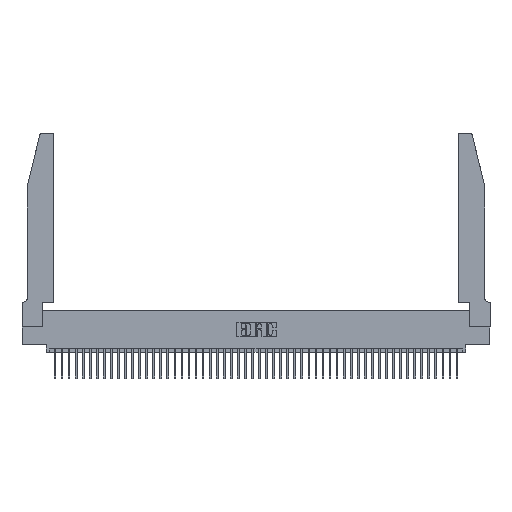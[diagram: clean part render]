
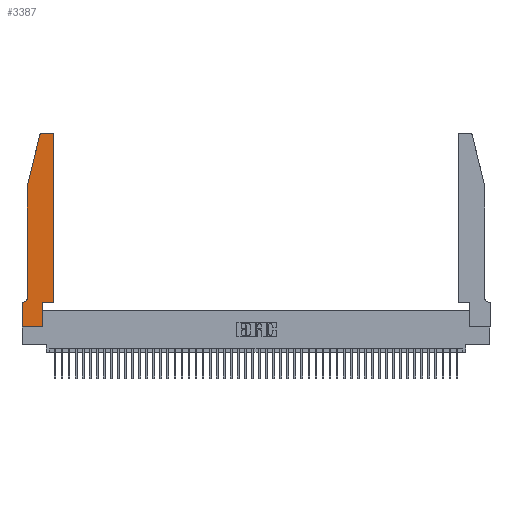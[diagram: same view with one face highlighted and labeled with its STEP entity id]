
A CAD part, top view. The second image highlights one B-rep face of the part: STEP entity #3387.
In plain terms, the highlighted planar face has unit normal (0, 0, 1).
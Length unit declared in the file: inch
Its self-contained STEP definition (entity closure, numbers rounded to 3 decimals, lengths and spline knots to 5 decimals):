
#514 = ORIENTED_EDGE ( 'NONE', *, *, #25352, .T. ) ;
#854 = VECTOR ( 'NONE', #18013, 39.37008 ) ;
#1100 = CARTESIAN_POINT ( 'NONE',  ( 0.0755, 0.42, 0.37 ) ) ;
#1218 = EDGE_CURVE ( 'NONE', #14511, #22834, #33169, .T. ) ;
#2102 = CARTESIAN_POINT ( 'NONE',  ( 0.0055, 0.35, 0.37 ) ) ;
#2210 = VERTEX_POINT ( 'NONE', #40274 ) ;
#2488 = LINE ( 'NONE', #4334, #41095 ) ;
#2883 = LINE ( 'NONE', #10523, #39128 ) ;
#2946 = CARTESIAN_POINT ( 'NONE',  ( 0., 0.35, 0.37 ) ) ;
#3387 = ADVANCED_FACE ( 'NONE', ( #33549 ), #14356, .T. ) ;
#3492 = EDGE_CURVE ( 'NONE', #10858, #14511, #30826, .T. ) ;
#4207 = ORIENTED_EDGE ( 'NONE', *, *, #3492, .T. ) ;
#4283 = CARTESIAN_POINT ( 'NONE',  ( 0.4505, 2.72, 0.37 ) ) ;
#4334 = CARTESIAN_POINT ( 'NONE',  ( 0., 0., 0.37 ) ) ;
#5247 = CARTESIAN_POINT ( 'NONE',  ( 0.284, 2.72, 0.37 ) ) ;
#6327 = CARTESIAN_POINT ( 'NONE',  ( 0.0755, 2., 0.37 ) ) ;
#7287 = ORIENTED_EDGE ( 'NONE', *, *, #33037, .T. ) ;
#8584 = AXIS2_PLACEMENT_3D ( 'NONE', #5247, #31466, #9052 ) ;
#9052 = DIRECTION ( 'NONE',  ( 1., 0., 0. ) ) ;
#10312 = CARTESIAN_POINT ( 'NONE',  ( 0., 0., 0.37 ) ) ;
#10523 = CARTESIAN_POINT ( 'NONE',  ( 0.4505, 0.35, 0.37 ) ) ;
#10858 = VERTEX_POINT ( 'NONE', #31291 ) ;
#11249 = CARTESIAN_POINT ( 'NONE',  ( 0.0755, 2., 0.37 ) ) ;
#11959 = DIRECTION ( 'NONE',  ( 0., -1., 0. ) ) ;
#12079 = ORIENTED_EDGE ( 'NONE', *, *, #45357, .T. ) ;
#12313 = CARTESIAN_POINT ( 'NONE',  ( 0., 0.35, 0.37 ) ) ;
#12674 = VECTOR ( 'NONE', #37459, 39.37008 ) ;
#13081 = AXIS2_PLACEMENT_3D ( 'NONE', #2946, #18090, #44031 ) ;
#13844 = LINE ( 'NONE', #11249, #12674 ) ;
#14031 = DIRECTION ( 'NONE',  ( 0., 1., 0. ) ) ;
#14294 = DIRECTION ( 'NONE',  ( 1., 0., 0. ) ) ;
#14356 = PLANE ( 'NONE',  #13081 ) ;
#14511 = VERTEX_POINT ( 'NONE', #16355 ) ;
#14753 = AXIS2_PLACEMENT_3D ( 'NONE', #43718, #21566, #47420 ) ;
#15510 = LINE ( 'NONE', #6327, #25458 ) ;
#16355 = CARTESIAN_POINT ( 'NONE',  ( 0.284, 2.75, 0.37 ) ) ;
#17189 = VERTEX_POINT ( 'NONE', #20565 ) ;
#17313 = DIRECTION ( 'NONE',  ( 0., 0., -1. ) ) ;
#17687 = ORIENTED_EDGE ( 'NONE', *, *, #45769, .T. ) ;
#18013 = DIRECTION ( 'NONE',  ( -1., 0., 0. ) ) ;
#18090 = DIRECTION ( 'NONE',  ( 0., 0., 1. ) ) ;
#18226 = VECTOR ( 'NONE', #14031, 39.37008 ) ;
#18697 = EDGE_CURVE ( 'NONE', #28160, #10858, #22471, .T. ) ;
#19185 = VERTEX_POINT ( 'NONE', #20687 ) ;
#19398 = LINE ( 'NONE', #43728, #18226 ) ;
#19445 = VERTEX_POINT ( 'NONE', #23279 ) ;
#19790 = ORIENTED_EDGE ( 'NONE', *, *, #20894, .T. ) ;
#20439 = EDGE_CURVE ( 'NONE', #2210, #17189, #19398, .T. ) ;
#20565 = CARTESIAN_POINT ( 'NONE',  ( 0.2865, 0.35, 0.37 ) ) ;
#20687 = CARTESIAN_POINT ( 'NONE',  ( 0.4505, 0.35, 0.37 ) ) ;
#20894 = EDGE_CURVE ( 'NONE', #17189, #19185, #2883, .T. ) ;
#21566 = DIRECTION ( 'NONE',  ( 0., 0., 1. ) ) ;
#22048 = ORIENTED_EDGE ( 'NONE', *, *, #18697, .T. ) ;
#22471 = CIRCLE ( 'NONE', #14753, 0.03 ) ;
#22691 = LINE ( 'NONE', #45994, #40075 ) ;
#22834 = VERTEX_POINT ( 'NONE', #40465 ) ;
#23279 = CARTESIAN_POINT ( 'NONE',  ( 0., 0., 0.37 ) ) ;
#23767 = EDGE_CURVE ( 'NONE', #35734, #32669, #22691, .T. ) ;
#23946 = EDGE_CURVE ( 'NONE', #24401, #35734, #25599, .T. ) ;
#24241 = EDGE_CURVE ( 'NONE', #22834, #43255, #13844, .T. ) ;
#24401 = VERTEX_POINT ( 'NONE', #1100 ) ;
#25139 = ORIENTED_EDGE ( 'NONE', *, *, #20439, .T. ) ;
#25352 = EDGE_CURVE ( 'NONE', #43255, #24401, #15510, .T. ) ;
#25458 = VECTOR ( 'NONE', #47146, 39.37008 ) ;
#25599 = CIRCLE ( 'NONE', #25849, 0.07 ) ;
#25849 = AXIS2_PLACEMENT_3D ( 'NONE', #39575, #17313, #43259 ) ;
#28125 = LINE ( 'NONE', #40066, #46545 ) ;
#28140 = CARTESIAN_POINT ( 'NONE',  ( 0.0755, 2., 0.37 ) ) ;
#28160 = VERTEX_POINT ( 'NONE', #4283 ) ;
#30825 = VECTOR ( 'NONE', #36591, 39.37008 ) ;
#30826 = LINE ( 'NONE', #47651, #854 ) ;
#31291 = CARTESIAN_POINT ( 'NONE',  ( 0.4205, 2.75, 0.37 ) ) ;
#31346 = ORIENTED_EDGE ( 'NONE', *, *, #1218, .T. ) ;
#31466 = DIRECTION ( 'NONE',  ( 0., 0., 1. ) ) ;
#32669 = VERTEX_POINT ( 'NONE', #12313 ) ;
#33037 = EDGE_CURVE ( 'NONE', #19445, #2210, #40658, .T. ) ;
#33169 = CIRCLE ( 'NONE', #8584, 0.03 ) ;
#33280 = EDGE_LOOP ( 'NONE', ( #4207, #31346, #47483, #514, #36483, #36989, #12079, #7287, #25139, #19790, #17687, #22048 ) ) ;
#33549 = FACE_OUTER_BOUND ( 'NONE', #33280, .T. ) ;
#35085 = DIRECTION ( 'NONE',  ( -1., 0., 0. ) ) ;
#35734 = VERTEX_POINT ( 'NONE', #2102 ) ;
#36483 = ORIENTED_EDGE ( 'NONE', *, *, #23946, .T. ) ;
#36591 = DIRECTION ( 'NONE',  ( 1., 0., 0. ) ) ;
#36989 = ORIENTED_EDGE ( 'NONE', *, *, #23767, .T. ) ;
#37459 = DIRECTION ( 'NONE',  ( -0.239, -0.971, 0. ) ) ;
#39128 = VECTOR ( 'NONE', #14294, 39.37008 ) ;
#39575 = CARTESIAN_POINT ( 'NONE',  ( 0.0055, 0.42, 0.37 ) ) ;
#40066 = CARTESIAN_POINT ( 'NONE',  ( 0.4505, 0.35, 0.37 ) ) ;
#40075 = VECTOR ( 'NONE', #35085, 39.37008 ) ;
#40274 = CARTESIAN_POINT ( 'NONE',  ( 0.2865, 0., 0.37 ) ) ;
#40465 = CARTESIAN_POINT ( 'NONE',  ( 0.25487, 2.72718, 0.37 ) ) ;
#40658 = LINE ( 'NONE', #10312, #30825 ) ;
#41095 = VECTOR ( 'NONE', #11959, 39.37008 ) ;
#43255 = VERTEX_POINT ( 'NONE', #28140 ) ;
#43259 = DIRECTION ( 'NONE',  ( -1., 0., 0. ) ) ;
#43718 = CARTESIAN_POINT ( 'NONE',  ( 0.4205, 2.72, 0.37 ) ) ;
#43728 = CARTESIAN_POINT ( 'NONE',  ( 0.2865, 0.35, 0.37 ) ) ;
#44031 = DIRECTION ( 'NONE',  ( 1., 0., 0. ) ) ;
#45357 = EDGE_CURVE ( 'NONE', #32669, #19445, #2488, .T. ) ;
#45769 = EDGE_CURVE ( 'NONE', #19185, #28160, #28125, .T. ) ;
#45994 = CARTESIAN_POINT ( 'NONE',  ( 0.0755, 0.35, 0.37 ) ) ;
#46545 = VECTOR ( 'NONE', #47438, 39.37008 ) ;
#47146 = DIRECTION ( 'NONE',  ( 0., -1., 0. ) ) ;
#47420 = DIRECTION ( 'NONE',  ( 1., 0., 0. ) ) ;
#47438 = DIRECTION ( 'NONE',  ( 0., 1., 0. ) ) ;
#47483 = ORIENTED_EDGE ( 'NONE', *, *, #24241, .T. ) ;
#47651 = CARTESIAN_POINT ( 'NONE',  ( 0.2605, 2.75, 0.37 ) ) ;
